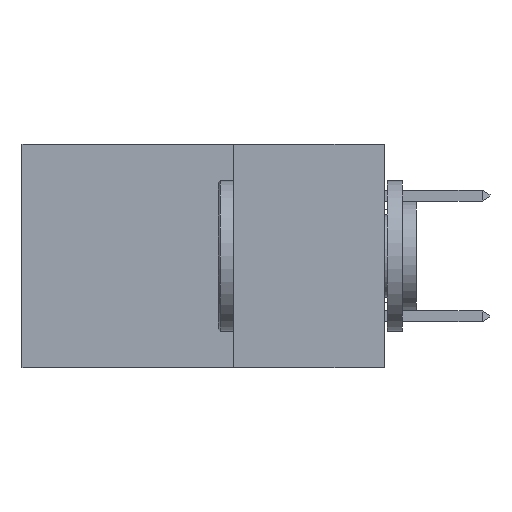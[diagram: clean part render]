
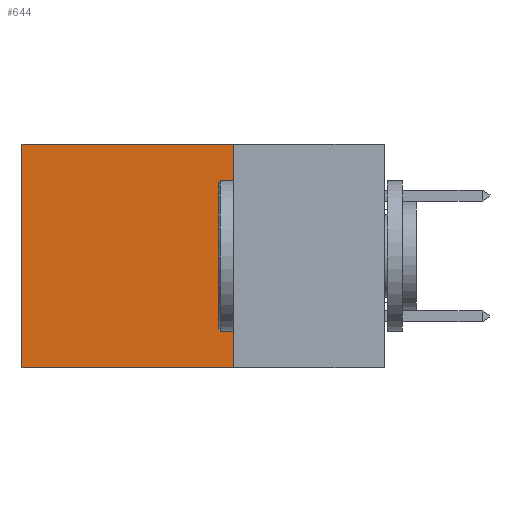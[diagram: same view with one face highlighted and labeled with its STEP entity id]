
A CAD part, left-side view. The second image highlights one B-rep face of the part: STEP entity #644.
In plain terms, the highlighted planar face has unit normal (-1, 0, 0).
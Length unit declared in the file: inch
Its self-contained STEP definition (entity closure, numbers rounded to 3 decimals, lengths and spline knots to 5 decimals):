
#57 = CARTESIAN_POINT ( 'NONE',  ( 0.2875, 0.25, 0. ) ) ;
#414 = ORIENTED_EDGE ( 'NONE', *, *, #9836, .F. ) ;
#644 = ADVANCED_FACE ( 'NONE', ( #3184 ), #1567, .F. ) ;
#772 = DIRECTION ( 'NONE',  ( 0., 0., -1. ) ) ;
#867 = VECTOR ( 'NONE', #8239, 39.37008 ) ;
#1003 = CARTESIAN_POINT ( 'NONE',  ( 0.2875, 0.6, 0. ) ) ;
#1310 = VERTEX_POINT ( 'NONE', #3940 ) ;
#1567 = PLANE ( 'NONE',  #3890 ) ;
#1797 = LINE ( 'NONE', #1003, #11185 ) ;
#2133 = VECTOR ( 'NONE', #4587, 39.37008 ) ;
#2431 = ORIENTED_EDGE ( 'NONE', *, *, #5436, .T. ) ;
#2443 = ORIENTED_EDGE ( 'NONE', *, *, #5162, .F. ) ;
#2448 = LINE ( 'NONE', #4530, #2133 ) ;
#2472 = CARTESIAN_POINT ( 'NONE',  ( 0.2875, 0.25, 0. ) ) ;
#2522 = ORIENTED_EDGE ( 'NONE', *, *, #4643, .T. ) ;
#2741 = VERTEX_POINT ( 'NONE', #6928 ) ;
#3184 = FACE_OUTER_BOUND ( 'NONE', #3408, .T. ) ;
#3408 = EDGE_LOOP ( 'NONE', ( #2431, #2443, #414, #2522 ) ) ;
#3810 = VERTEX_POINT ( 'NONE', #10376 ) ;
#3890 = AXIS2_PLACEMENT_3D ( 'NONE', #2472, #3986, #10377 ) ;
#3940 = CARTESIAN_POINT ( 'NONE',  ( 0.2875, 0.25, 0. ) ) ;
#3986 = DIRECTION ( 'NONE',  ( 1., 0., 0. ) ) ;
#4530 = CARTESIAN_POINT ( 'NONE',  ( 0.2875, 0.25, -0.37 ) ) ;
#4587 = DIRECTION ( 'NONE',  ( 0., 1., 0. ) ) ;
#4643 = EDGE_CURVE ( 'NONE', #1310, #9762, #11069, .T. ) ;
#5162 = EDGE_CURVE ( 'NONE', #2741, #3810, #2448, .T. ) ;
#5436 = EDGE_CURVE ( 'NONE', #9762, #3810, #1797, .T. ) ;
#6928 = CARTESIAN_POINT ( 'NONE',  ( 0.2875, 0.25, -0.37 ) ) ;
#7210 = CARTESIAN_POINT ( 'NONE',  ( 0.2875, 0.6, 0. ) ) ;
#8239 = DIRECTION ( 'NONE',  ( 0., 0., -1. ) ) ;
#8989 = VECTOR ( 'NONE', #12281, 39.37008 ) ;
#9762 = VERTEX_POINT ( 'NONE', #7210 ) ;
#9836 = EDGE_CURVE ( 'NONE', #1310, #2741, #10990, .T. ) ;
#10377 = DIRECTION ( 'NONE',  ( 0., 0., -1. ) ) ;
#10376 = CARTESIAN_POINT ( 'NONE',  ( 0.2875, 0.6, -0.37 ) ) ;
#10990 = LINE ( 'NONE', #57, #867 ) ;
#11069 = LINE ( 'NONE', #12201, #8989 ) ;
#11185 = VECTOR ( 'NONE', #772, 39.37008 ) ;
#12201 = CARTESIAN_POINT ( 'NONE',  ( 0.2875, 0.25, 0. ) ) ;
#12281 = DIRECTION ( 'NONE',  ( 0., 1., 0. ) ) ;
